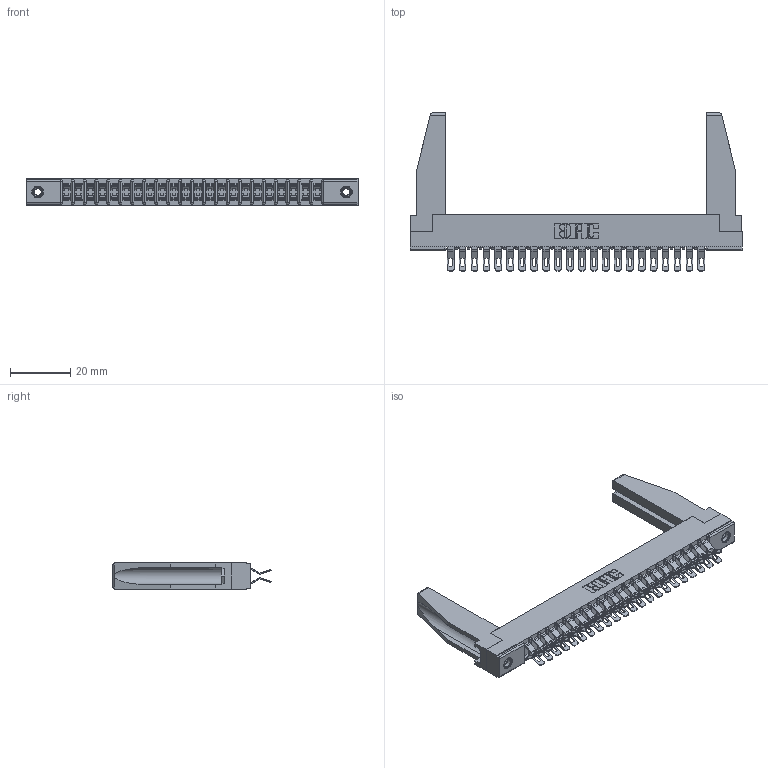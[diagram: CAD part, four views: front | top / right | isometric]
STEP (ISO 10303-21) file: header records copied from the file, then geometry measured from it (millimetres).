
FILE_DESCRIPTION (( 'STEP AP203' ), '1' );
FILE_NAME ('357-044-455-278.STEP', '2020-10-04T00:24:46', ( '' ), ( '' ), 'SwSTEP 2.0', 'SolidWorks 2020', '' );
FILE_SCHEMA (( 'CONFIG_CONTROL_DESIGN' ));
Length unit declared in the file: inch
Products named in the file (5): 357-044-455-278; 307-220-078; 307 Part_.156 Dia Mounting Holes; 345-250-001_345-250-001-102; 307-290-001_555
Assembly tree (49 placements, depth 2):
  357-044-455-278
    307 Part_.156 Dia Mounting Holes
    307-290-001_555  x44
    307-220-078  x2
    345-250-001_345-250-001-102  x2
Bounding box: 110.19 x 52.45 x 8.71 mm (x, y, z)
Volume: 11331.7 mm3; surface area: 17509.5 mm2
Topology: 49 solids, 49 shells, 2955 faces, 8617 edges, 5614 vertices
Faces by surface type: plane 1650, cylinder 1243, sphere 46, cone 12, torus 4
Entity records: 25006 total; most frequent: CARTESIAN_POINT 4112, ORIENTED_EDGE 4034, DIRECTION 3997, EDGE_CURVE 2017, LINE 1531, VECTOR 1531, VERTEX_POINT 1306, AXIS2_PLACEMENT_3D 1233
